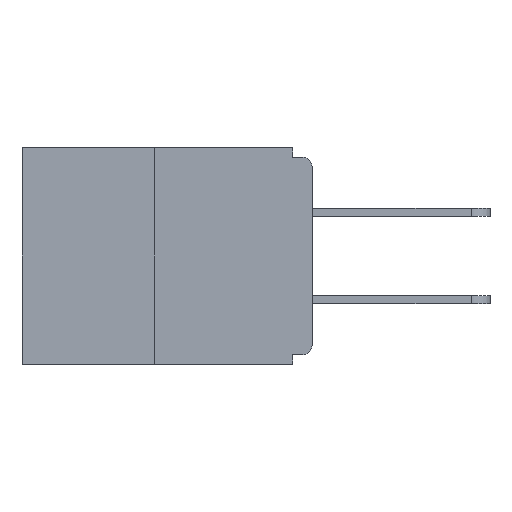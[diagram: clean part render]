
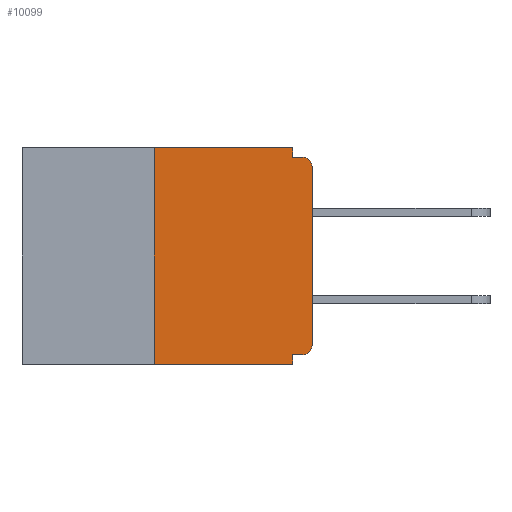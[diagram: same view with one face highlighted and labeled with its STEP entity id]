
A CAD part, left-side view. The second image highlights one B-rep face of the part: STEP entity #10099.
In plain terms, the highlighted planar face has unit normal (-1, 0, 0).
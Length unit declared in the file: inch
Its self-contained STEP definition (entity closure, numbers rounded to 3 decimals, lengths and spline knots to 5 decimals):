
#50 = CARTESIAN_POINT ( 'NONE',  ( 0., 0.015, -0.313 ) ) ;
#652 = VECTOR ( 'NONE', #22131, 39.37008 ) ;
#734 = VECTOR ( 'NONE', #24133, 39.37008 ) ;
#885 = DIRECTION ( 'NONE',  ( 1., 0., 0. ) ) ;
#893 = EDGE_CURVE ( 'NONE', #8140, #25645, #19616, .T. ) ;
#1895 = CIRCLE ( 'NONE', #11493, 0.015 ) ;
#2214 = ORIENTED_EDGE ( 'NONE', *, *, #9243, .F. ) ;
#2358 = VERTEX_POINT ( 'NONE', #11551 ) ;
#2542 = EDGE_CURVE ( 'NONE', #18988, #8487, #1895, .T. ) ;
#3460 = CARTESIAN_POINT ( 'NONE',  ( 0., 0., -0.03 ) ) ;
#6215 = EDGE_LOOP ( 'NONE', ( #15069, #16089, #10314, #21029, #2214, #11016, #21039, #23832, #25032, #24307 ) ) ;
#6442 = CARTESIAN_POINT ( 'NONE',  ( 0., 0.031, -0.343 ) ) ;
#6606 = FACE_OUTER_BOUND ( 'NONE', #6215, .T. ) ;
#6774 = PLANE ( 'NONE',  #15945 ) ;
#7092 = CARTESIAN_POINT ( 'NONE',  ( 0., 0.015, -0.03 ) ) ;
#7335 = CARTESIAN_POINT ( 'NONE',  ( 0., 0.46, -0.343 ) ) ;
#7467 = LINE ( 'NONE', #21697, #13588 ) ;
#7724 = CARTESIAN_POINT ( 'NONE',  ( 0., 0., 0. ) ) ;
#8140 = VERTEX_POINT ( 'NONE', #17954 ) ;
#8419 = DIRECTION ( 'NONE',  ( 0., 0., 1. ) ) ;
#8474 = DIRECTION ( 'NONE',  ( 0., 0., -1. ) ) ;
#8487 = VERTEX_POINT ( 'NONE', #19838 ) ;
#9243 = EDGE_CURVE ( 'NONE', #18988, #19130, #7467, .T. ) ;
#9262 = CARTESIAN_POINT ( 'NONE',  ( 0., 0.015, -0.328 ) ) ;
#10099 = ADVANCED_FACE ( 'NONE', ( #6606 ), #6774, .F. ) ;
#10245 = CARTESIAN_POINT ( 'NONE',  ( 0., 0.25, -0.343 ) ) ;
#10314 = ORIENTED_EDGE ( 'NONE', *, *, #12091, .T. ) ;
#10375 = CARTESIAN_POINT ( 'NONE',  ( 0., 0.031, -0.343 ) ) ;
#11016 = ORIENTED_EDGE ( 'NONE', *, *, #2542, .T. ) ;
#11083 = VECTOR ( 'NONE', #16242, 39.37008 ) ;
#11251 = DIRECTION ( 'NONE',  ( 0., 0., -1. ) ) ;
#11493 = AXIS2_PLACEMENT_3D ( 'NONE', #50, #20824, #8474 ) ;
#11533 = DIRECTION ( 'NONE',  ( 0., -1., 0. ) ) ;
#11551 = CARTESIAN_POINT ( 'NONE',  ( 0., 0.031, -0.015 ) ) ;
#11698 = CIRCLE ( 'NONE', #24512, 0.015 ) ;
#12091 = EDGE_CURVE ( 'NONE', #15145, #13714, #17110, .T. ) ;
#12866 = VECTOR ( 'NONE', #11533, 39.37008 ) ;
#13192 = CARTESIAN_POINT ( 'NONE',  ( 0., 0.46, 0. ) ) ;
#13588 = VECTOR ( 'NONE', #13684, 39.37008 ) ;
#13684 = DIRECTION ( 'NONE',  ( 0., 1., 0. ) ) ;
#13686 = CARTESIAN_POINT ( 'NONE',  ( 0., 0.46, 0. ) ) ;
#13714 = VERTEX_POINT ( 'NONE', #6442 ) ;
#14779 = DIRECTION ( 'NONE',  ( 0., 0., -1. ) ) ;
#15069 = ORIENTED_EDGE ( 'NONE', *, *, #893, .F. ) ;
#15145 = VERTEX_POINT ( 'NONE', #10245 ) ;
#15658 = EDGE_CURVE ( 'NONE', #2358, #23120, #15892, .T. ) ;
#15892 = LINE ( 'NONE', #26560, #11083 ) ;
#15945 = AXIS2_PLACEMENT_3D ( 'NONE', #13192, #885, #21200 ) ;
#16086 = LINE ( 'NONE', #7724, #652 ) ;
#16089 = ORIENTED_EDGE ( 'NONE', *, *, #24481, .F. ) ;
#16242 = DIRECTION ( 'NONE',  ( 0., -1., 0. ) ) ;
#17110 = LINE ( 'NONE', #7335, #734 ) ;
#17180 = CARTESIAN_POINT ( 'NONE',  ( 0., 0.031, 0. ) ) ;
#17954 = CARTESIAN_POINT ( 'NONE',  ( 0., 0.25, 0. ) ) ;
#18988 = VERTEX_POINT ( 'NONE', #9262 ) ;
#19130 = VERTEX_POINT ( 'NONE', #22043 ) ;
#19280 = VECTOR ( 'NONE', #14779, 39.37008 ) ;
#19616 = LINE ( 'NONE', #13686, #12866 ) ;
#19838 = CARTESIAN_POINT ( 'NONE',  ( 0., 0., -0.313 ) ) ;
#20761 = CARTESIAN_POINT ( 'NONE',  ( 0., 0.031, 0. ) ) ;
#20824 = DIRECTION ( 'NONE',  ( -1., 0., 0. ) ) ;
#21026 = CARTESIAN_POINT ( 'NONE',  ( 0., 0.25, 0. ) ) ;
#21029 = ORIENTED_EDGE ( 'NONE', *, *, #22346, .F. ) ;
#21039 = ORIENTED_EDGE ( 'NONE', *, *, #23272, .T. ) ;
#21200 = DIRECTION ( 'NONE',  ( 0., 0., -1. ) ) ;
#21257 = DIRECTION ( 'NONE',  ( 0., 0., -1. ) ) ;
#21677 = DIRECTION ( 'NONE',  ( -1., 0., 0. ) ) ;
#21697 = CARTESIAN_POINT ( 'NONE',  ( 0., 0., -0.328 ) ) ;
#21826 = EDGE_CURVE ( 'NONE', #25645, #2358, #22384, .T. ) ;
#22043 = CARTESIAN_POINT ( 'NONE',  ( 0., 0.031, -0.328 ) ) ;
#22131 = DIRECTION ( 'NONE',  ( 0., 0., 1. ) ) ;
#22346 = EDGE_CURVE ( 'NONE', #19130, #13714, #25150, .T. ) ;
#22384 = LINE ( 'NONE', #17180, #24016 ) ;
#23120 = VERTEX_POINT ( 'NONE', #25846 ) ;
#23272 = EDGE_CURVE ( 'NONE', #8487, #26535, #16086, .T. ) ;
#23767 = VECTOR ( 'NONE', #8419, 39.37008 ) ;
#23832 = ORIENTED_EDGE ( 'NONE', *, *, #26464, .T. ) ;
#24016 = VECTOR ( 'NONE', #21257, 39.37008 ) ;
#24133 = DIRECTION ( 'NONE',  ( 0., -1., 0. ) ) ;
#24307 = ORIENTED_EDGE ( 'NONE', *, *, #21826, .F. ) ;
#24481 = EDGE_CURVE ( 'NONE', #15145, #8140, #25702, .T. ) ;
#24512 = AXIS2_PLACEMENT_3D ( 'NONE', #7092, #21677, #11251 ) ;
#25032 = ORIENTED_EDGE ( 'NONE', *, *, #15658, .F. ) ;
#25150 = LINE ( 'NONE', #10375, #19280 ) ;
#25645 = VERTEX_POINT ( 'NONE', #20761 ) ;
#25702 = LINE ( 'NONE', #21026, #23767 ) ;
#25846 = CARTESIAN_POINT ( 'NONE',  ( 0., 0.015, -0.015 ) ) ;
#26464 = EDGE_CURVE ( 'NONE', #26535, #23120, #11698, .T. ) ;
#26535 = VERTEX_POINT ( 'NONE', #3460 ) ;
#26560 = CARTESIAN_POINT ( 'NONE',  ( 0., 0., -0.015 ) ) ;
